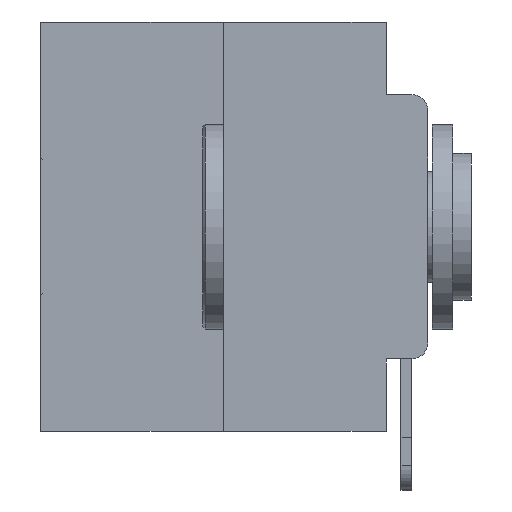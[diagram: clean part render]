
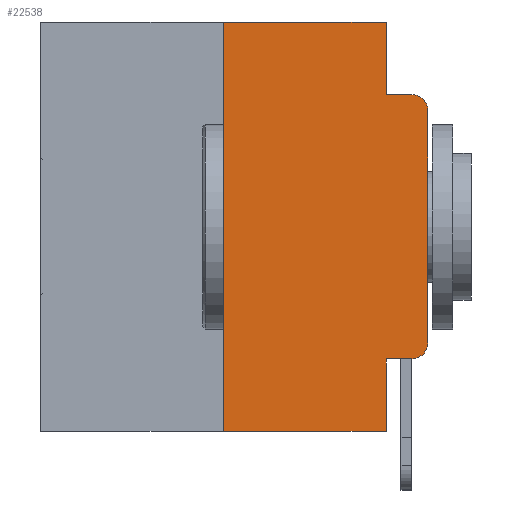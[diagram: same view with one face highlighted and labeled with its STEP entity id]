
A CAD part, left-side view. The second image highlights one B-rep face of the part: STEP entity #22538.
In plain terms, the highlighted planar face has unit normal (-1, 0, 0).
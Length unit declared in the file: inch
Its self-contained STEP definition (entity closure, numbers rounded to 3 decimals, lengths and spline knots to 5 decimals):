
#9 = CARTESIAN_POINT ( 'NONE',  ( 0., 0.02, -0.3915 ) ) ;
#366 = ORIENTED_EDGE ( 'NONE', *, *, #5639, .F. ) ;
#1214 = VECTOR ( 'NONE', #8799, 39.37008 ) ;
#1719 = VERTEX_POINT ( 'NONE', #16496 ) ;
#1953 = LINE ( 'NONE', #6410, #1214 ) ;
#2050 = CARTESIAN_POINT ( 'NONE',  ( 0., 0.051, -0.4115 ) ) ;
#2295 = PLANE ( 'NONE',  #4472 ) ;
#2363 = EDGE_LOOP ( 'NONE', ( #10835, #5974, #20028, #30544, #366, #14556, #3043, #7525, #27698, #8649 ) ) ;
#2454 = DIRECTION ( 'NONE',  ( 0., 0., -1. ) ) ;
#3043 = ORIENTED_EDGE ( 'NONE', *, *, #8907, .T. ) ;
#3095 = VERTEX_POINT ( 'NONE', #7867 ) ;
#3169 = LINE ( 'NONE', #6898, #15068 ) ;
#3756 = CARTESIAN_POINT ( 'NONE',  ( 0., 0.051, 0. ) ) ;
#4472 = AXIS2_PLACEMENT_3D ( 'NONE', #18883, #4728, #21229 ) ;
#4627 = VERTEX_POINT ( 'NONE', #22894 ) ;
#4728 = DIRECTION ( 'NONE',  ( 1., 0., 0. ) ) ;
#5012 = CARTESIAN_POINT ( 'NONE',  ( 0., 0.051, -0.0885 ) ) ;
#5639 = EDGE_CURVE ( 'NONE', #14260, #23490, #8397, .T. ) ;
#5974 = ORIENTED_EDGE ( 'NONE', *, *, #7516, .T. ) ;
#6045 = EDGE_CURVE ( 'NONE', #4627, #18255, #16134, .T. ) ;
#6285 = LINE ( 'NONE', #3756, #13370 ) ;
#6390 = VERTEX_POINT ( 'NONE', #15917 ) ;
#6410 = CARTESIAN_POINT ( 'NONE',  ( 0., 0.473, -0.5 ) ) ;
#6898 = CARTESIAN_POINT ( 'NONE',  ( 0., 0.051, 0. ) ) ;
#7516 = EDGE_CURVE ( 'NONE', #18255, #1719, #14722, .T. ) ;
#7525 = ORIENTED_EDGE ( 'NONE', *, *, #27856, .F. ) ;
#7867 = CARTESIAN_POINT ( 'NONE',  ( 0., 0.02, -0.4115 ) ) ;
#8397 = LINE ( 'NONE', #15562, #20201 ) ;
#8411 = DIRECTION ( 'NONE',  ( -1., 0., 0. ) ) ;
#8649 = ORIENTED_EDGE ( 'NONE', *, *, #11819, .T. ) ;
#8799 = DIRECTION ( 'NONE',  ( 0., -1., 0. ) ) ;
#8907 = EDGE_CURVE ( 'NONE', #16390, #22998, #1953, .T. ) ;
#9049 = EDGE_CURVE ( 'NONE', #16559, #1719, #9417, .T. ) ;
#9110 = CARTESIAN_POINT ( 'NONE',  ( 0., 0., -0.1085 ) ) ;
#9277 = DIRECTION ( 'NONE',  ( 0., 0., -1. ) ) ;
#9417 = LINE ( 'NONE', #28155, #28120 ) ;
#10835 = ORIENTED_EDGE ( 'NONE', *, *, #6045, .T. ) ;
#10957 = DIRECTION ( 'NONE',  ( 0., 0., -1. ) ) ;
#11819 = EDGE_CURVE ( 'NONE', #3095, #4627, #20001, .T. ) ;
#12361 = DIRECTION ( 'NONE',  ( 0., 0., 1. ) ) ;
#12848 = EDGE_CURVE ( 'NONE', #23490, #16559, #3169, .T. ) ;
#12955 = AXIS2_PLACEMENT_3D ( 'NONE', #22518, #8411, #24824 ) ;
#13370 = VECTOR ( 'NONE', #10957, 39.37008 ) ;
#14260 = VERTEX_POINT ( 'NONE', #27451 ) ;
#14556 = ORIENTED_EDGE ( 'NONE', *, *, #24156, .F. ) ;
#14722 = CIRCLE ( 'NONE', #12955, 0.02 ) ;
#15000 = VECTOR ( 'NONE', #18560, 39.37008 ) ;
#15068 = VECTOR ( 'NONE', #9277, 39.37008 ) ;
#15405 = VECTOR ( 'NONE', #12361, 39.37008 ) ;
#15562 = CARTESIAN_POINT ( 'NONE',  ( 0., 0.473, 0. ) ) ;
#15917 = CARTESIAN_POINT ( 'NONE',  ( 0., 0.051, -0.4115 ) ) ;
#16134 = LINE ( 'NONE', #23989, #15405 ) ;
#16390 = VERTEX_POINT ( 'NONE', #24069 ) ;
#16464 = LINE ( 'NONE', #2050, #15000 ) ;
#16496 = CARTESIAN_POINT ( 'NONE',  ( 0., 0.02, -0.0885 ) ) ;
#16559 = VERTEX_POINT ( 'NONE', #5012 ) ;
#16670 = DIRECTION ( 'NONE',  ( -1., 0., 0. ) ) ;
#16719 = DIRECTION ( 'NONE',  ( 0., 0., 1. ) ) ;
#17923 = DIRECTION ( 'NONE',  ( 0., -1., 0. ) ) ;
#18255 = VERTEX_POINT ( 'NONE', #9110 ) ;
#18345 = CARTESIAN_POINT ( 'NONE',  ( 0., 0.051, -0.5 ) ) ;
#18560 = DIRECTION ( 'NONE',  ( 0., -1., 0. ) ) ;
#18883 = CARTESIAN_POINT ( 'NONE',  ( 0., 0.473, 0. ) ) ;
#20001 = CIRCLE ( 'NONE', #25134, 0.02 ) ;
#20028 = ORIENTED_EDGE ( 'NONE', *, *, #9049, .F. ) ;
#20201 = VECTOR ( 'NONE', #17923, 39.37008 ) ;
#20362 = CARTESIAN_POINT ( 'NONE',  ( 0., 0.051, 0. ) ) ;
#21082 = FACE_OUTER_BOUND ( 'NONE', #2363, .T. ) ;
#21229 = DIRECTION ( 'NONE',  ( 0., 0., -1. ) ) ;
#22518 = CARTESIAN_POINT ( 'NONE',  ( 0., 0.02, -0.1085 ) ) ;
#22538 = ADVANCED_FACE ( 'NONE', ( #21082 ), #2295, .F. ) ;
#22894 = CARTESIAN_POINT ( 'NONE',  ( 0., 0., -0.3915 ) ) ;
#22998 = VERTEX_POINT ( 'NONE', #18345 ) ;
#23490 = VERTEX_POINT ( 'NONE', #20362 ) ;
#23989 = CARTESIAN_POINT ( 'NONE',  ( 0., 0., 0. ) ) ;
#24069 = CARTESIAN_POINT ( 'NONE',  ( 0., 0.25, -0.5 ) ) ;
#24156 = EDGE_CURVE ( 'NONE', #16390, #14260, #27858, .T. ) ;
#24824 = DIRECTION ( 'NONE',  ( 0., 0., -1. ) ) ;
#25134 = AXIS2_PLACEMENT_3D ( 'NONE', #9, #16670, #2454 ) ;
#27133 = VECTOR ( 'NONE', #16719, 39.37008 ) ;
#27451 = CARTESIAN_POINT ( 'NONE',  ( 0., 0.25, 0. ) ) ;
#27698 = ORIENTED_EDGE ( 'NONE', *, *, #30552, .T. ) ;
#27856 = EDGE_CURVE ( 'NONE', #6390, #22998, #6285, .T. ) ;
#27858 = LINE ( 'NONE', #30542, #27133 ) ;
#28120 = VECTOR ( 'NONE', #30475, 39.37008 ) ;
#28155 = CARTESIAN_POINT ( 'NONE',  ( 0., 0.051, -0.0885 ) ) ;
#30475 = DIRECTION ( 'NONE',  ( 0., -1., 0. ) ) ;
#30542 = CARTESIAN_POINT ( 'NONE',  ( 0., 0.25, 0. ) ) ;
#30544 = ORIENTED_EDGE ( 'NONE', *, *, #12848, .F. ) ;
#30552 = EDGE_CURVE ( 'NONE', #6390, #3095, #16464, .T. ) ;
